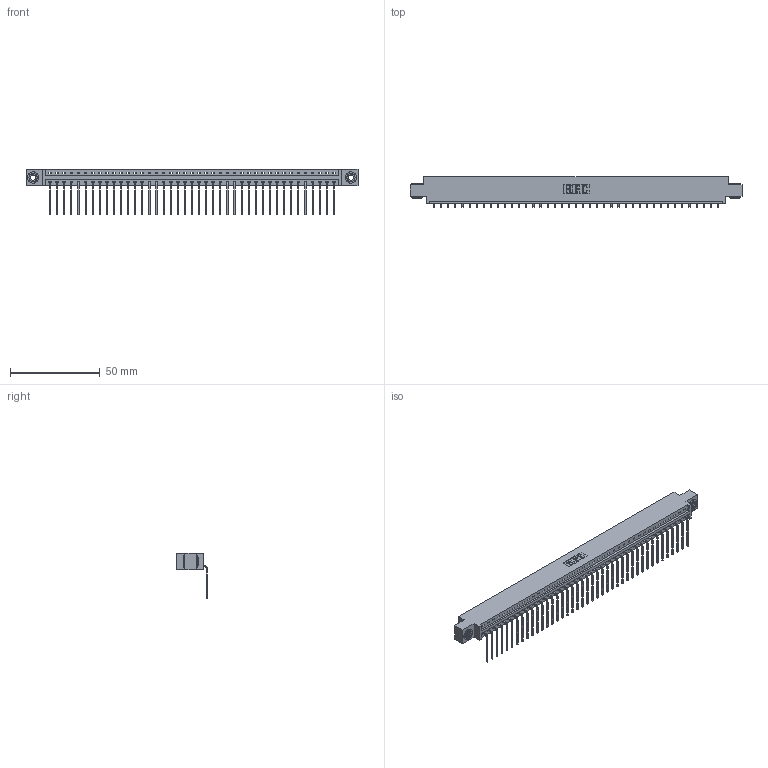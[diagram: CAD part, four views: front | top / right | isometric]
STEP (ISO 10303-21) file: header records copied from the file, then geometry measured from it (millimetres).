
FILE_DESCRIPTION (( 'STEP AP203' ), '1' );
FILE_NAME ('387-041-559-603.STEP', '2019-10-04T20:20:24', ( '' ), ( '' ), 'SwSTEP 2.0', 'SolidWorks 2016', '' );
FILE_SCHEMA (( 'CONFIG_CONTROL_DESIGN' ));
Length unit declared in the file: inch
Products named in the file (4): 345-292-001_558 559 Tail - 1; 387-041-559-603; 337 Part_0.170 Offset - 0.156 Dia-TH; 345-250-002_345-250-002-102
Assembly tree (44 placements, depth 2):
  387-041-559-603
    337 Part_0.170 Offset - 0.156 Dia-TH
    345-292-001_558 559 Tail - 1  x41
    345-250-002_345-250-002-102  x2
Bounding box: 185.47 x 17.09 x 25.53 mm (x, y, z)
Volume: 19302.6 mm3; surface area: 21109.1 mm2
Topology: 44 solids, 44 shells, 2780 faces, 8353 edges, 5510 vertices
Faces by surface type: plane 2052, cylinder 720, cone 8
Entity records: 31472 total; most frequent: CARTESIAN_POINT 5460, ORIENTED_EDGE 5430, DIRECTION 4631, EDGE_CURVE 2715, VECTOR 2563, LINE 2563, VERTEX_POINT 1806, AXIS2_PLACEMENT_3D 1034
